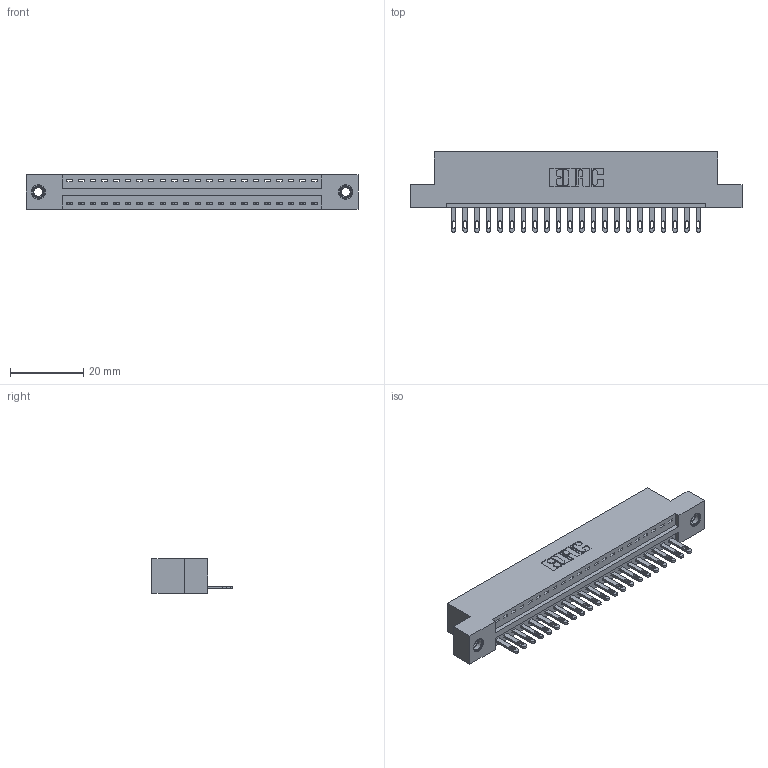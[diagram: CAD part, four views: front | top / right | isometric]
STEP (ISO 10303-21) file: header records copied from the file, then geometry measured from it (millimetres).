
FILE_DESCRIPTION (( 'STEP AP203' ), '1' );
FILE_NAME ('896-022-500-107.STEP', '2021-07-27T16:55:37', ( '' ), ( '' ), 'SwSTEP 2.0', 'SolidWorks 2020', '' );
FILE_SCHEMA (( 'CONFIG_CONTROL_DESIGN' ));
Length unit declared in the file: inch
Products named in the file (4): 846 Part_Flush Mounting Lugs - 0.156 Dia-TI; 345-250-001_345-250-005-103; 345-292-001_345-293-100; 896-022-500-107
Assembly tree (25 placements, depth 2):
  896-022-500-107
    846 Part_Flush Mounting Lugs - 0.156 Dia-TI
    345-292-001_345-293-100  x22
    345-250-001_345-250-005-103  x2
Bounding box: 90.42 x 21.84 x 9.4 mm (x, y, z)
Volume: 8517.9 mm3; surface area: 10516.3 mm2
Topology: 25 solids, 25 shells, 1370 faces, 4161 edges, 2766 vertices
Faces by surface type: plane 856, cylinder 498, cone 12, torus 4
Entity records: 17462 total; most frequent: CARTESIAN_POINT 2981, ORIENTED_EDGE 2930, DIRECTION 2683, EDGE_CURVE 1465, VECTOR 1221, LINE 1221, VERTEX_POINT 972, AXIS2_PLACEMENT_3D 731
